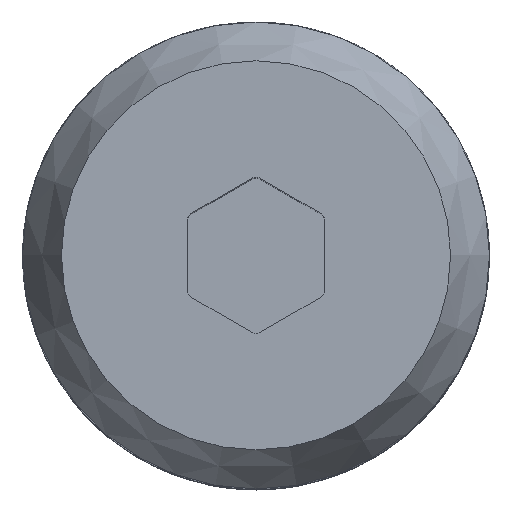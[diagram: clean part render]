
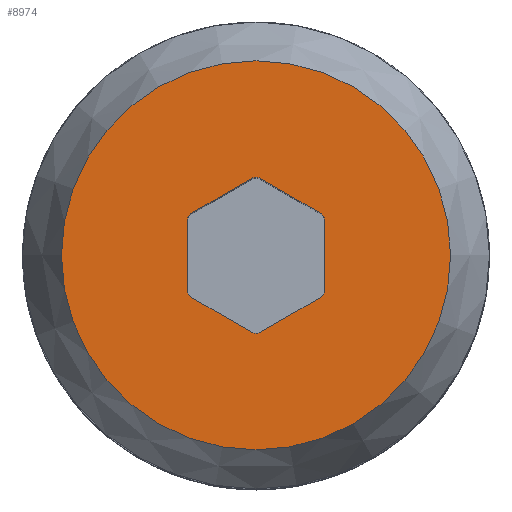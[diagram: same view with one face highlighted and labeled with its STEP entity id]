
A CAD part, top view. The second image highlights one B-rep face of the part: STEP entity #8974.
In plain terms, the highlighted planar face has unit normal (0, 0, 1).
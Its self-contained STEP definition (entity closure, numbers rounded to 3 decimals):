
#275=PLANE('',#9554);
#537=FACE_BOUND('',#1771,.T.);
#1167=FACE_OUTER_BOUND('',#1770,.T.);
#1770=EDGE_LOOP('',(#6668));
#1771=EDGE_LOOP('',(#6669,#6670,#6671,#6672,#6673,#6674,#6675,#6676,#6677,
#6678,#6679,#6680));
#2464=LINE('',#13034,#3226);
#2465=LINE('',#13038,#3227);
#2466=LINE('',#13042,#3228);
#2467=LINE('',#13046,#3229);
#2468=LINE('',#13050,#3230);
#2469=LINE('',#13053,#3231);
#3226=VECTOR('',#10102,10.);
#3227=VECTOR('',#10105,10.);
#3228=VECTOR('',#10108,10.);
#3229=VECTOR('',#10111,10.);
#3230=VECTOR('',#10114,10.);
#3231=VECTOR('',#10117,10.);
#3827=CIRCLE('',#9521,7.5);
#3859=CIRCLE('',#9555,0.35);
#3860=CIRCLE('',#9556,0.35);
#3861=CIRCLE('',#9557,0.35);
#3862=CIRCLE('',#9558,0.35);
#3863=CIRCLE('',#9559,0.35);
#3864=CIRCLE('',#9560,0.35);
#3900=VERTEX_POINT('',#11327);
#4352=VERTEX_POINT('',#13030);
#4353=VERTEX_POINT('',#13031);
#4354=VERTEX_POINT('',#13033);
#4355=VERTEX_POINT('',#13035);
#4356=VERTEX_POINT('',#13037);
#4357=VERTEX_POINT('',#13039);
#4358=VERTEX_POINT('',#13041);
#4359=VERTEX_POINT('',#13043);
#4360=VERTEX_POINT('',#13045);
#4361=VERTEX_POINT('',#13047);
#4362=VERTEX_POINT('',#13049);
#4363=VERTEX_POINT('',#13051);
#4821=EDGE_CURVE('',#3900,#3900,#3827,.T.);
#5278=EDGE_CURVE('',#4352,#4353,#3859,.T.);
#5279=EDGE_CURVE('',#4353,#4354,#2464,.T.);
#5280=EDGE_CURVE('',#4354,#4355,#3860,.T.);
#5281=EDGE_CURVE('',#4355,#4356,#2465,.T.);
#5282=EDGE_CURVE('',#4356,#4357,#3861,.T.);
#5283=EDGE_CURVE('',#4357,#4358,#2466,.T.);
#5284=EDGE_CURVE('',#4358,#4359,#3862,.T.);
#5285=EDGE_CURVE('',#4359,#4360,#2467,.T.);
#5286=EDGE_CURVE('',#4360,#4361,#3863,.T.);
#5287=EDGE_CURVE('',#4361,#4362,#2468,.T.);
#5288=EDGE_CURVE('',#4362,#4363,#3864,.T.);
#5289=EDGE_CURVE('',#4363,#4352,#2469,.T.);
#6668=ORIENTED_EDGE('',*,*,#4821,.F.);
#6669=ORIENTED_EDGE('',*,*,#5278,.T.);
#6670=ORIENTED_EDGE('',*,*,#5279,.T.);
#6671=ORIENTED_EDGE('',*,*,#5280,.T.);
#6672=ORIENTED_EDGE('',*,*,#5281,.T.);
#6673=ORIENTED_EDGE('',*,*,#5282,.T.);
#6674=ORIENTED_EDGE('',*,*,#5283,.T.);
#6675=ORIENTED_EDGE('',*,*,#5284,.T.);
#6676=ORIENTED_EDGE('',*,*,#5285,.T.);
#6677=ORIENTED_EDGE('',*,*,#5286,.T.);
#6678=ORIENTED_EDGE('',*,*,#5287,.T.);
#6679=ORIENTED_EDGE('',*,*,#5288,.T.);
#6680=ORIENTED_EDGE('',*,*,#5289,.T.);
#8974=ADVANCED_FACE('',(#1167,#537),#275,.F.);
#9521=AXIS2_PLACEMENT_3D('',#11328,#9871,#9872);
#9554=AXIS2_PLACEMENT_3D('',#13029,#10098,#10099);
#9555=AXIS2_PLACEMENT_3D('',#13032,#10100,#10101);
#9556=AXIS2_PLACEMENT_3D('',#13036,#10103,#10104);
#9557=AXIS2_PLACEMENT_3D('',#13040,#10106,#10107);
#9558=AXIS2_PLACEMENT_3D('',#13044,#10109,#10110);
#9559=AXIS2_PLACEMENT_3D('',#13048,#10112,#10113);
#9560=AXIS2_PLACEMENT_3D('',#13052,#10115,#10116);
#9871=DIRECTION('center_axis',(0.,0.,
-1.));
#9872=DIRECTION('ref_axis',(-1.,0.,0.));
#10098=DIRECTION('center_axis',(0.,0.,
-1.));
#10099=DIRECTION('ref_axis',(1.,0.,0.));
#10100=DIRECTION('center_axis',(0.,0.,
-1.));
#10101=DIRECTION('ref_axis',(0.5,-0.866,0.));
#10102=DIRECTION('',(-0.866,0.5,0.));
#10103=DIRECTION('center_axis',(0.,0.,
-1.));
#10104=DIRECTION('ref_axis',(-0.5,-0.866,0.));
#10105=DIRECTION('',(0.,1.,0.));
#10106=DIRECTION('center_axis',(0.,0.,
-1.));
#10107=DIRECTION('ref_axis',(-1.,0.,0.));
#10108=DIRECTION('',(0.866,0.5,0.));
#10109=DIRECTION('center_axis',(0.,0.,
-1.));
#10110=DIRECTION('ref_axis',(-0.5,0.866,0.));
#10111=DIRECTION('',(0.866,-0.5,0.));
#10112=DIRECTION('center_axis',(0.,0.,
-1.));
#10113=DIRECTION('ref_axis',(0.5,0.866,0.));
#10114=DIRECTION('',(0.,-1.,0.));
#10115=DIRECTION('center_axis',(0.,0.,
-1.));
#10116=DIRECTION('ref_axis',(1.,0.,0.));
#10117=DIRECTION('',(-0.866,-0.5,0.));
#11327=CARTESIAN_POINT('',(211.743,205.136,-42.067));
#11328=CARTESIAN_POINT('Origin',(204.243,205.136,-42.067));
#13029=CARTESIAN_POINT('Origin',(204.243,205.136,-42.067));
#13030=CARTESIAN_POINT('',(204.418,202.177,-42.067));
#13031=CARTESIAN_POINT('',(204.068,202.177,-42.067));
#13032=CARTESIAN_POINT('Origin',(204.243,202.48,-42.067));
#13033=CARTESIAN_POINT('',(201.768,203.505,-42.067));
#13034=CARTESIAN_POINT('',(204.068,202.177,-42.067));
#13035=CARTESIAN_POINT('',(201.593,203.808,-42.067));
#13036=CARTESIAN_POINT('Origin',(201.943,203.808,-42.067));
#13037=CARTESIAN_POINT('',(201.593,206.464,-42.067));
#13038=CARTESIAN_POINT('',(201.593,203.808,-42.067));
#13039=CARTESIAN_POINT('',(201.768,206.767,-42.067));
#13040=CARTESIAN_POINT('Origin',(201.943,206.464,-42.067));
#13041=CARTESIAN_POINT('',(204.068,208.095,-42.067));
#13042=CARTESIAN_POINT('',(201.768,206.767,-42.067));
#13043=CARTESIAN_POINT('',(204.418,208.095,-42.067));
#13044=CARTESIAN_POINT('Origin',(204.243,207.791,-42.067));
#13045=CARTESIAN_POINT('',(206.718,206.767,-42.067));
#13046=CARTESIAN_POINT('',(204.418,208.095,-42.067));
#13047=CARTESIAN_POINT('',(206.893,206.464,-42.067));
#13048=CARTESIAN_POINT('Origin',(206.543,206.464,-42.067));
#13049=CARTESIAN_POINT('',(206.893,203.808,-42.067));
#13050=CARTESIAN_POINT('',(206.893,206.464,-42.067));
#13051=CARTESIAN_POINT('',(206.718,203.505,-42.067));
#13052=CARTESIAN_POINT('Origin',(206.543,203.808,-42.067));
#13053=CARTESIAN_POINT('',(206.718,203.505,-42.067));
